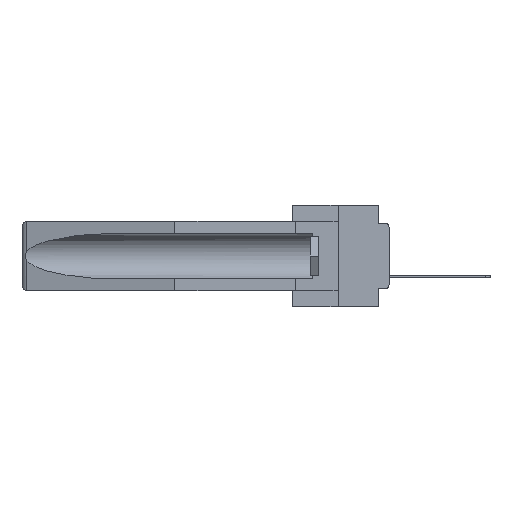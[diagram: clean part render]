
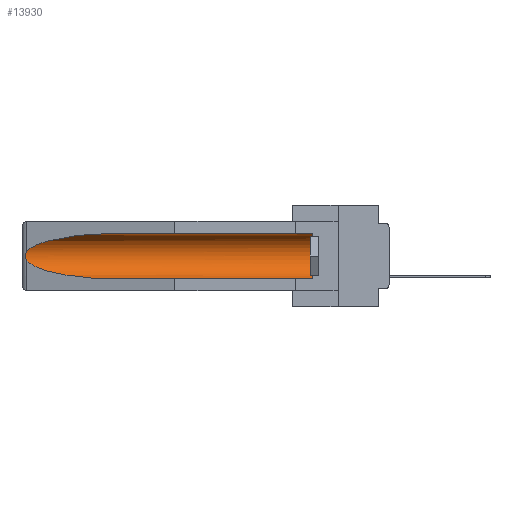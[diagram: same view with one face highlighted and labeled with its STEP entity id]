
A CAD part, left-side view. The second image highlights one B-rep face of the part: STEP entity #13930.
In plain terms, the highlighted cylindrical face has radius 2.857 mm (diameter 5.715 mm), a partial arc.
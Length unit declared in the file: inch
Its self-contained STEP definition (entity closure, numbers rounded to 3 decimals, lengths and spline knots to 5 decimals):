
#228 = CARTESIAN_POINT ( 'NONE',  ( 0.26537, 1.52718, -0.19328 ) ) ;
#1610 = CARTESIAN_POINT ( 'NONE',  ( 0.26537, 1.52718, -0.19328 ) ) ;
#1652 = ORIENTED_EDGE ( 'NONE', *, *, #15594, .T. ) ;
#1901 = DIRECTION ( 'NONE',  ( 0., 1., 0. ) ) ;
#2407 = CIRCLE ( 'NONE', #21608, 0.1125 ) ;
#2486 = CARTESIAN_POINT ( 'NONE',  ( 0.155, 1.07973, -0.284 ) ) ;
#2562 = DIRECTION ( 'NONE',  ( 0., 1., 0. ) ) ;
#2717 = CARTESIAN_POINT ( 'NONE',  ( 0.21114, 1.30732, -0.059 ) ) ;
#2721 = CYLINDRICAL_SURFACE ( 'NONE', #30336, 0.1125 ) ;
#2983 = ORIENTED_EDGE ( 'NONE', *, *, #11692, .T. ) ;
#3686 = CARTESIAN_POINT ( 'NONE',  ( 0.155, 1.07973, -0.284 ) ) ;
#3897 =( BOUNDED_CURVE ( )  B_SPLINE_CURVE ( 3, ( #21427, #25857, #16830, #2486 ),
 .UNSPECIFIED., .F., .F. ) 
 B_SPLINE_CURVE_WITH_KNOTS ( ( 4, 4 ),
 ( 0.1948, 1.5708 ),
 .UNSPECIFIED. ) 
 CURVE ( )  GEOMETRIC_REPRESENTATION_ITEM ( )  RATIONAL_B_SPLINE_CURVE ( ( 1., 0.848, 0.848, 1. ) ) 
 REPRESENTATION_ITEM ( '' )  );
#4855 = CARTESIAN_POINT ( 'NONE',  ( 0.2673, 1.53269, -0.17917 ) ) ;
#5352 = CARTESIAN_POINT ( 'NONE',  ( 0.25451, 1.48313, -0.09465 ) ) ;
#6455 = CARTESIAN_POINT ( 'NONE',  ( 0.26655, 1.53094, -0.18657 ) ) ;
#6569 = EDGE_CURVE ( 'NONE', #14221, #22580, #3897, .T. ) ;
#6609 = CARTESIAN_POINT ( 'NONE',  ( 0.155, -0.30754, -0.059 ) ) ;
#6703 = VERTEX_POINT ( 'NONE', #10044 ) ;
#6809 = ORIENTED_EDGE ( 'NONE', *, *, #25522, .T. ) ;
#7308 = CARTESIAN_POINT ( 'NONE',  ( 0.155, 1.07973, -0.059 ) ) ;
#8759 = LINE ( 'NONE', #6609, #9857 ) ;
#8847 = CARTESIAN_POINT ( 'NONE',  ( 0.155, -0.30754, -0.284 ) ) ;
#9002 = LINE ( 'NONE', #8847, #12838 ) ;
#9487 = CARTESIAN_POINT ( 'NONE',  ( 0.2673, 1.5327, -0.16383 ) ) ;
#9857 = VECTOR ( 'NONE', #11367, 39.37008 ) ;
#10044 = CARTESIAN_POINT ( 'NONE',  ( 0.26537, 1.52718, -0.14972 ) ) ;
#10417 = ORIENTED_EDGE ( 'NONE', *, *, #15071, .T. ) ;
#11367 = DIRECTION ( 'NONE',  ( 0., 1., 0. ) ) ;
#11692 = EDGE_CURVE ( 'NONE', #6703, #14221, #20233, .T. ) ;
#11790 = CARTESIAN_POINT ( 'NONE',  ( 0.26597, 1.52961, -0.15275 ) ) ;
#11956 = CARTESIAN_POINT ( 'NONE',  ( 0.26537, 1.52718, -0.14972 ) ) ;
#12127 = CARTESIAN_POINT ( 'NONE',  ( 0.26537, 1.52718, -0.14972 ) ) ;
#12822 = DIRECTION ( 'NONE',  ( 0., -1., 0. ) ) ;
#12838 = VECTOR ( 'NONE', #1901, 39.37008 ) ;
#13490 = ORIENTED_EDGE ( 'NONE', *, *, #6569, .T. ) ;
#13930 = ADVANCED_FACE ( 'NONE', ( #16450 ), #2721, .F. ) ;
#14015 = ORIENTED_EDGE ( 'NONE', *, *, #16294, .F. ) ;
#14221 = VERTEX_POINT ( 'NONE', #1610 ) ;
#14406 = VERTEX_POINT ( 'NONE', #7308 ) ;
#15071 = EDGE_CURVE ( 'NONE', #18412, #28833, #2407, .T. ) ;
#15285 = DIRECTION ( 'NONE',  ( 0., 0., 1. ) ) ;
#15594 = EDGE_CURVE ( 'NONE', #28833, #14406, #8759, .T. ) ;
#16294 = EDGE_CURVE ( 'NONE', #18412, #22580, #9002, .T. ) ;
#16450 = FACE_OUTER_BOUND ( 'NONE', #24071, .T. ) ;
#16830 = CARTESIAN_POINT ( 'NONE',  ( 0.21114, 1.30732, -0.284 ) ) ;
#17059 = CARTESIAN_POINT ( 'NONE',  ( 0.155, 1.07973, -0.059 ) ) ;
#18412 = VERTEX_POINT ( 'NONE', #20330 ) ;
#18888 = CARTESIAN_POINT ( 'NONE',  ( 0.2675, 1.53308, -0.16763 ) ) ;
#18911 = CARTESIAN_POINT ( 'NONE',  ( 0.155, -0.30754, -0.1715 ) ) ;
#19486 = CARTESIAN_POINT ( 'NONE',  ( 0.155, 0.126, -0.059 ) ) ;
#20233 = B_SPLINE_CURVE_WITH_KNOTS ( 'NONE', 3,
 ( #11956, #11790, #21180, #9487, #18888, #28208, #4855, #6455, #28363, #228 ),
 .UNSPECIFIED., .F., .F.,
 ( 4, 2, 2, 2, 4 ),
 ( 0., 0.00029, 0.00058, 0.00087, 0.00117 ),
 .UNSPECIFIED. ) ;
#20330 = CARTESIAN_POINT ( 'NONE',  ( 0.155, 0.126, -0.284 ) ) ;
#21180 = CARTESIAN_POINT ( 'NONE',  ( 0.26654, 1.53092, -0.15636 ) ) ;
#21427 = CARTESIAN_POINT ( 'NONE',  ( 0.26537, 1.52718, -0.19328 ) ) ;
#21608 = AXIS2_PLACEMENT_3D ( 'NONE', #27532, #12822, #15285 ) ;
#22580 = VERTEX_POINT ( 'NONE', #3686 ) ;
#22966 =( BOUNDED_CURVE ( )  B_SPLINE_CURVE ( 3, ( #17059, #2717, #5352, #12127 ),
 .UNSPECIFIED., .F., .F. ) 
 B_SPLINE_CURVE_WITH_KNOTS ( ( 4, 4 ),
 ( 4.71239, 6.08839 ),
 .UNSPECIFIED. ) 
 CURVE ( )  GEOMETRIC_REPRESENTATION_ITEM ( )  RATIONAL_B_SPLINE_CURVE ( ( 1., 0.848, 0.848, 1. ) ) 
 REPRESENTATION_ITEM ( '' )  );
#24071 = EDGE_LOOP ( 'NONE', ( #6809, #2983, #13490, #14015, #10417, #1652 ) ) ;
#25522 = EDGE_CURVE ( 'NONE', #14406, #6703, #22966, .T. ) ;
#25857 = CARTESIAN_POINT ( 'NONE',  ( 0.25451, 1.48313, -0.24835 ) ) ;
#27532 = CARTESIAN_POINT ( 'NONE',  ( 0.155, 0.126, -0.1715 ) ) ;
#28084 = DIRECTION ( 'NONE',  ( 0., 0., 1. ) ) ;
#28208 = CARTESIAN_POINT ( 'NONE',  ( 0.2675, 1.53308, -0.17534 ) ) ;
#28363 = CARTESIAN_POINT ( 'NONE',  ( 0.26597, 1.5296, -0.19026 ) ) ;
#28833 = VERTEX_POINT ( 'NONE', #19486 ) ;
#30336 = AXIS2_PLACEMENT_3D ( 'NONE', #18911, #2562, #28084 ) ;
